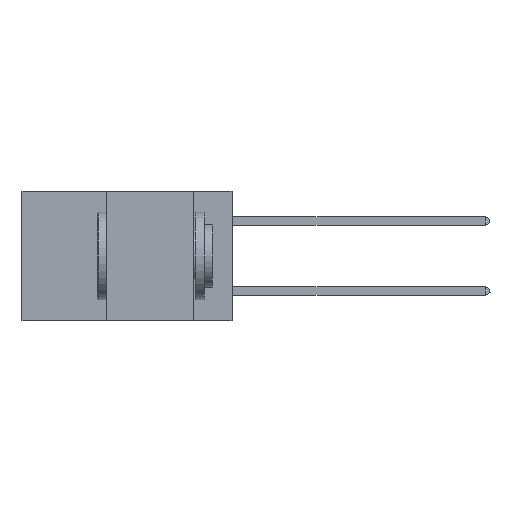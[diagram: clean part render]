
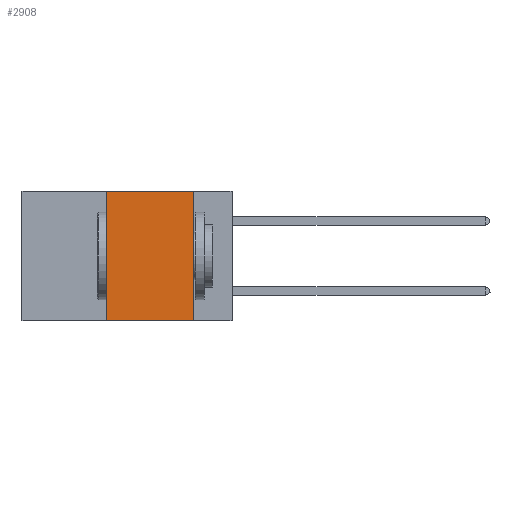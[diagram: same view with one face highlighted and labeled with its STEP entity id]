
A CAD part, left-side view. The second image highlights one B-rep face of the part: STEP entity #2908.
In plain terms, the highlighted planar face has unit normal (-1, 0, 0).
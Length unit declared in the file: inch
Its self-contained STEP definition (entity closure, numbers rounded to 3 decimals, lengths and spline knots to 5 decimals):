
#740 = DIRECTION ( 'NONE',  ( 0., -1., 0. ) ) ;
#755 = CARTESIAN_POINT ( 'NONE',  ( 0., 0.6, 0. ) ) ;
#776 = VERTEX_POINT ( 'NONE', #5960 ) ;
#1293 = VECTOR ( 'NONE', #8608, 39.37008 ) ;
#1302 = LINE ( 'NONE', #8188, #8623 ) ;
#1943 = DIRECTION ( 'NONE',  ( 0., -1., 0. ) ) ;
#1986 = LINE ( 'NONE', #7684, #1293 ) ;
#2588 = CARTESIAN_POINT ( 'NONE',  ( 0., 0.11, -0.37 ) ) ;
#2908 = ADVANCED_FACE ( 'NONE', ( #11771 ), #6246, .F. ) ;
#3068 = DIRECTION ( 'NONE',  ( 0., 0., -1. ) ) ;
#4128 = EDGE_CURVE ( 'NONE', #4762, #7538, #10583, .T. ) ;
#4762 = VERTEX_POINT ( 'NONE', #8654 ) ;
#4857 = DIRECTION ( 'NONE',  ( 1., 0., 0. ) ) ;
#4944 = ORIENTED_EDGE ( 'NONE', *, *, #11575, .T. ) ;
#5960 = CARTESIAN_POINT ( 'NONE',  ( 0., 0.36, -0.37 ) ) ;
#6036 = CARTESIAN_POINT ( 'NONE',  ( 0., 0.36, 0. ) ) ;
#6246 = PLANE ( 'NONE',  #11880 ) ;
#7538 = VERTEX_POINT ( 'NONE', #9941 ) ;
#7684 = CARTESIAN_POINT ( 'NONE',  ( 0., 0.11, 0. ) ) ;
#8059 = CARTESIAN_POINT ( 'NONE',  ( 0., 0.6, 0. ) ) ;
#8188 = CARTESIAN_POINT ( 'NONE',  ( 0., 0.6, -0.37 ) ) ;
#8608 = DIRECTION ( 'NONE',  ( 0., 0., -1. ) ) ;
#8623 = VECTOR ( 'NONE', #1943, 39.37008 ) ;
#8654 = CARTESIAN_POINT ( 'NONE',  ( 0., 0.36, 0. ) ) ;
#9941 = CARTESIAN_POINT ( 'NONE',  ( 0., 0.11, 0. ) ) ;
#10051 = ORIENTED_EDGE ( 'NONE', *, *, #12811, .F. ) ;
#10583 = LINE ( 'NONE', #755, #11147 ) ;
#10714 = DIRECTION ( 'NONE',  ( 0., 0., 1. ) ) ;
#11051 = ORIENTED_EDGE ( 'NONE', *, *, #12205, .F. ) ;
#11147 = VECTOR ( 'NONE', #740, 39.37008 ) ;
#11218 = VERTEX_POINT ( 'NONE', #2588 ) ;
#11526 = EDGE_LOOP ( 'NONE', ( #10051, #12910, #11051, #4944 ) ) ;
#11575 = EDGE_CURVE ( 'NONE', #776, #11218, #1302, .T. ) ;
#11771 = FACE_OUTER_BOUND ( 'NONE', #11526, .T. ) ;
#11880 = AXIS2_PLACEMENT_3D ( 'NONE', #8059, #4857, #3068 ) ;
#12205 = EDGE_CURVE ( 'NONE', #776, #4762, #12903, .T. ) ;
#12642 = VECTOR ( 'NONE', #10714, 39.37008 ) ;
#12811 = EDGE_CURVE ( 'NONE', #7538, #11218, #1986, .T. ) ;
#12903 = LINE ( 'NONE', #6036, #12642 ) ;
#12910 = ORIENTED_EDGE ( 'NONE', *, *, #4128, .F. ) ;
